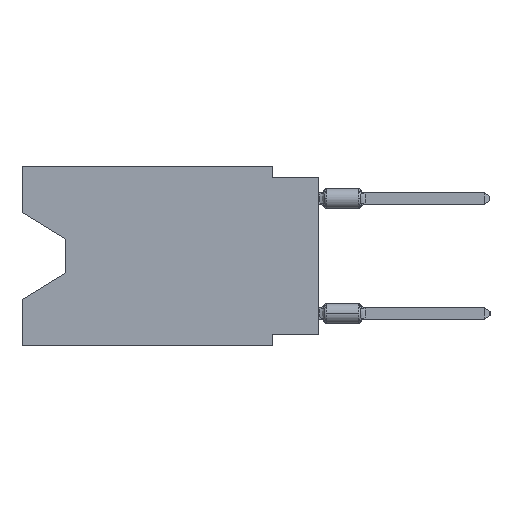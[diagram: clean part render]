
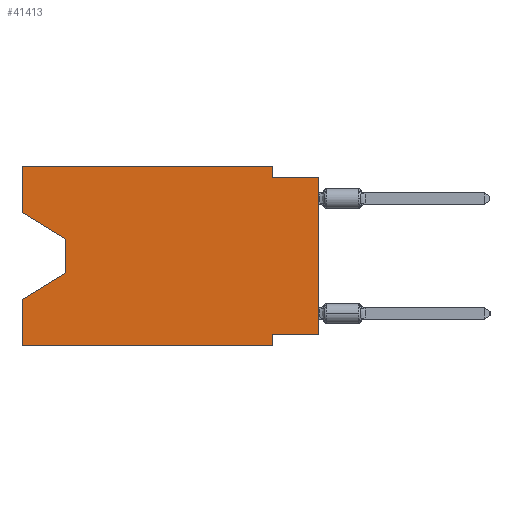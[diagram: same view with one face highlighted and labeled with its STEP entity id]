
A CAD part, left-side view. The second image highlights one B-rep face of the part: STEP entity #41413.
In plain terms, the highlighted planar face has unit normal (-1, 0, 0).
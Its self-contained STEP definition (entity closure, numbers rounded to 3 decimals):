
#168 = VERTEX_POINT ( 'NONE', #7749 ) ;
#1341 = LINE ( 'NONE', #30553, #58338 ) ;
#2994 = LINE ( 'NONE', #35663, #35025 ) ;
#3164 = VERTEX_POINT ( 'NONE', #11576 ) ;
#3728 = ORIENTED_EDGE ( 'NONE', *, *, #51633, .T. ) ;
#4614 = CARTESIAN_POINT ( 'NONE',  ( 0., 2.54, 0. ) ) ;
#4816 = LINE ( 'NONE', #9548, #15341 ) ;
#4872 = CARTESIAN_POINT ( 'NONE',  ( 0., 0., -0.635 ) ) ;
#7749 = CARTESIAN_POINT ( 'NONE',  ( 0., 0., -0.635 ) ) ;
#7773 = LINE ( 'NONE', #14271, #59630 ) ;
#8253 = CARTESIAN_POINT ( 'NONE',  ( 0., 2.54, 0. ) ) ;
#8667 = DIRECTION ( 'NONE',  ( 0., -1., 0. ) ) ;
#8760 = CARTESIAN_POINT ( 'NONE',  ( 0., 16.383, 0. ) ) ;
#9548 = CARTESIAN_POINT ( 'NONE',  ( 0., 16.383, 0. ) ) ;
#9690 = DIRECTION ( 'NONE',  ( 1., 0., 0. ) ) ;
#9719 = DIRECTION ( 'NONE',  ( 0., 1., 0. ) ) ;
#9747 = AXIS2_PLACEMENT_3D ( 'NONE', #8760, #9690, #28258 ) ;
#10299 = VECTOR ( 'NONE', #25470, 1000. ) ;
#10964 = CARTESIAN_POINT ( 'NONE',  ( 0., 13.97, -4.013 ) ) ;
#11152 = CARTESIAN_POINT ( 'NONE',  ( 0., 2.54, -9.906 ) ) ;
#11576 = CARTESIAN_POINT ( 'NONE',  ( 0., 16.383, 0. ) ) ;
#11923 = LINE ( 'NONE', #30184, #10299 ) ;
#12117 = ORIENTED_EDGE ( 'NONE', *, *, #21258, .T. ) ;
#13219 = CARTESIAN_POINT ( 'NONE',  ( 0., 0., -9.271 ) ) ;
#13817 = VERTEX_POINT ( 'NONE', #13219 ) ;
#14059 = VECTOR ( 'NONE', #32364, 1000. ) ;
#14125 = VERTEX_POINT ( 'NONE', #21006 ) ;
#14271 = CARTESIAN_POINT ( 'NONE',  ( 0., 16.383, -9.906 ) ) ;
#15341 = VECTOR ( 'NONE', #61320, 1000. ) ;
#16162 = LINE ( 'NONE', #11152, #53774 ) ;
#16763 = DIRECTION ( 'NONE',  ( 0., 0., -1. ) ) ;
#16928 = CARTESIAN_POINT ( 'NONE',  ( 0., 16.383, 0. ) ) ;
#19046 = CARTESIAN_POINT ( 'NONE',  ( 0., 2.54, -0.635 ) ) ;
#21006 = CARTESIAN_POINT ( 'NONE',  ( 0., 2.54, -9.271 ) ) ;
#21085 = ORIENTED_EDGE ( 'NONE', *, *, #60412, .F. ) ;
#21201 = VECTOR ( 'NONE', #32456, 1000. ) ;
#21258 = EDGE_CURVE ( 'NONE', #36798, #36633, #7773, .T. ) ;
#21628 = DIRECTION ( 'NONE',  ( 0., 0., 1. ) ) ;
#22322 = CARTESIAN_POINT ( 'NONE',  ( 0., 13.97, -5.893 ) ) ;
#22333 = EDGE_CURVE ( 'NONE', #13817, #14125, #29204, .T. ) ;
#22429 = CARTESIAN_POINT ( 'NONE',  ( 0., 16.383, -9.906 ) ) ;
#22741 = VERTEX_POINT ( 'NONE', #4614 ) ;
#22939 = CARTESIAN_POINT ( 'NONE',  ( 0., 16.383, -2.546 ) ) ;
#25470 = DIRECTION ( 'NONE',  ( 0., 0., -1. ) ) ;
#26096 = ORIENTED_EDGE ( 'NONE', *, *, #52888, .T. ) ;
#26785 = LINE ( 'NONE', #8253, #60165 ) ;
#26876 = DIRECTION ( 'NONE',  ( 0., -1., 0. ) ) ;
#27585 = VERTEX_POINT ( 'NONE', #10964 ) ;
#27849 = CARTESIAN_POINT ( 'NONE',  ( 0., 2.54, -9.906 ) ) ;
#28080 = CARTESIAN_POINT ( 'NONE',  ( 0., 0., 0. ) ) ;
#28258 = DIRECTION ( 'NONE',  ( 0., 0., -1. ) ) ;
#28392 = LINE ( 'NONE', #28080, #21201 ) ;
#28726 = DIRECTION ( 'NONE',  ( 0., -1., 0. ) ) ;
#29204 = LINE ( 'NONE', #43895, #44589 ) ;
#29399 = VERTEX_POINT ( 'NONE', #39732 ) ;
#30184 = CARTESIAN_POINT ( 'NONE',  ( 0., 13.97, -4.013 ) ) ;
#30553 = CARTESIAN_POINT ( 'NONE',  ( 0., 16.383, -2.546 ) ) ;
#30749 = ORIENTED_EDGE ( 'NONE', *, *, #22333, .F. ) ;
#31120 = EDGE_CURVE ( 'NONE', #22741, #39181, #26785, .T. ) ;
#31183 = DIRECTION ( 'NONE',  ( 0., 0., -1. ) ) ;
#32364 = DIRECTION ( 'NONE',  ( 0., 0.855, -0.519 ) ) ;
#32456 = DIRECTION ( 'NONE',  ( 0., 0., 1. ) ) ;
#35025 = VECTOR ( 'NONE', #26876, 1000. ) ;
#35069 = EDGE_CURVE ( 'NONE', #46695, #27585, #1341, .T. ) ;
#35663 = CARTESIAN_POINT ( 'NONE',  ( 0., 16.383, 0. ) ) ;
#36633 = VERTEX_POINT ( 'NONE', #27849 ) ;
#36798 = VERTEX_POINT ( 'NONE', #22429 ) ;
#38263 = EDGE_CURVE ( 'NONE', #36798, #41856, #4816, .T. ) ;
#39181 = VERTEX_POINT ( 'NONE', #19046 ) ;
#39732 = CARTESIAN_POINT ( 'NONE',  ( 0., 13.97, -5.893 ) ) ;
#40039 = EDGE_CURVE ( 'NONE', #46695, #3164, #61149, .T. ) ;
#40925 = EDGE_CURVE ( 'NONE', #14125, #36633, #16162, .T. ) ;
#41413 = ADVANCED_FACE ( 'NONE', ( #61157 ), #52667, .F. ) ;
#41464 = LINE ( 'NONE', #22322, #14059 ) ;
#41856 = VERTEX_POINT ( 'NONE', #61694 ) ;
#42171 = ORIENTED_EDGE ( 'NONE', *, *, #46333, .F. ) ;
#43295 = ORIENTED_EDGE ( 'NONE', *, *, #40039, .F. ) ;
#43895 = CARTESIAN_POINT ( 'NONE',  ( 0., 0., -9.271 ) ) ;
#44589 = VECTOR ( 'NONE', #9719, 1000. ) ;
#46333 = EDGE_CURVE ( 'NONE', #3164, #22741, #2994, .T. ) ;
#46601 = ORIENTED_EDGE ( 'NONE', *, *, #35069, .T. ) ;
#46695 = VERTEX_POINT ( 'NONE', #22939 ) ;
#48556 = ORIENTED_EDGE ( 'NONE', *, *, #38263, .F. ) ;
#49162 = EDGE_CURVE ( 'NONE', #29399, #41856, #41464, .T. ) ;
#51633 = EDGE_CURVE ( 'NONE', #13817, #168, #28392, .T. ) ;
#52279 = LINE ( 'NONE', #4872, #55981 ) ;
#52667 = PLANE ( 'NONE',  #9747 ) ;
#52888 = EDGE_CURVE ( 'NONE', #27585, #29399, #11923, .T. ) ;
#53735 = VECTOR ( 'NONE', #21628, 1000. ) ;
#53774 = VECTOR ( 'NONE', #16763, 1000. ) ;
#54386 = DIRECTION ( 'NONE',  ( 0., -0.855, -0.519 ) ) ;
#55100 = ORIENTED_EDGE ( 'NONE', *, *, #49162, .T. ) ;
#55981 = VECTOR ( 'NONE', #8667, 1000. ) ;
#57079 = ORIENTED_EDGE ( 'NONE', *, *, #31120, .F. ) ;
#58338 = VECTOR ( 'NONE', #54386, 1000. ) ;
#59330 = EDGE_LOOP ( 'NONE', ( #46601, #26096, #55100, #48556, #12117, #59607, #30749, #3728, #21085, #57079, #42171, #43295 ) ) ;
#59607 = ORIENTED_EDGE ( 'NONE', *, *, #40925, .F. ) ;
#59630 = VECTOR ( 'NONE', #28726, 1000. ) ;
#60165 = VECTOR ( 'NONE', #31183, 1000. ) ;
#60412 = EDGE_CURVE ( 'NONE', #39181, #168, #52279, .T. ) ;
#61149 = LINE ( 'NONE', #16928, #53735 ) ;
#61157 = FACE_OUTER_BOUND ( 'NONE', #59330, .T. ) ;
#61320 = DIRECTION ( 'NONE',  ( 0., 0., 1. ) ) ;
#61694 = CARTESIAN_POINT ( 'NONE',  ( 0., 16.383, -7.36 ) ) ;
